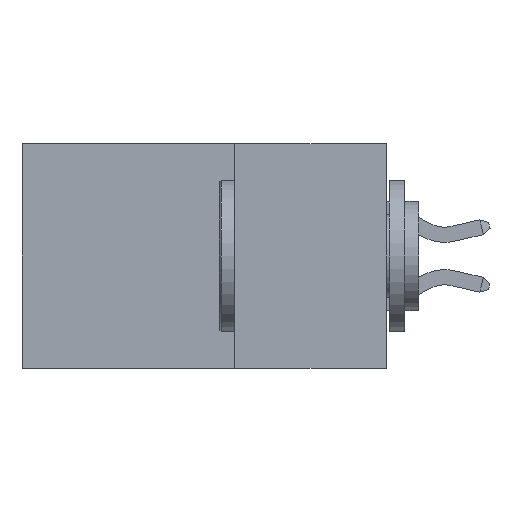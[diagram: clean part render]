
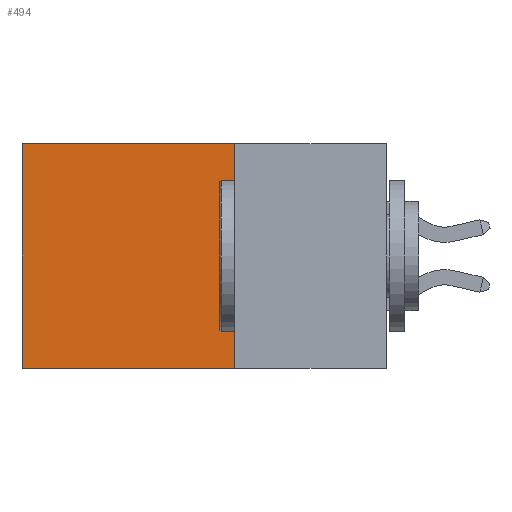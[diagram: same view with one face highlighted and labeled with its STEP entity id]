
A CAD part, left-side view. The second image highlights one B-rep face of the part: STEP entity #494.
In plain terms, the highlighted planar face has unit normal (-1, 0, 0).
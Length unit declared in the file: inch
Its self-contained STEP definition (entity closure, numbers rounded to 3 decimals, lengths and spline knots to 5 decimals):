
#291 = VECTOR ( 'NONE', #782, 39.37008 ) ;
#494 = ADVANCED_FACE ( 'NONE', ( #12663 ), #8164, .F. ) ;
#782 = DIRECTION ( 'NONE',  ( 0., 1., 0. ) ) ;
#1333 = VECTOR ( 'NONE', #10145, 39.37008 ) ;
#1853 = CARTESIAN_POINT ( 'NONE',  ( 0.298, 0.25, -0.37 ) ) ;
#2065 = VECTOR ( 'NONE', #10781, 39.37008 ) ;
#2215 = CARTESIAN_POINT ( 'NONE',  ( 0.298, 0.6, 0. ) ) ;
#2294 = EDGE_CURVE ( 'NONE', #17666, #16864, #17444, .T. ) ;
#3424 = CARTESIAN_POINT ( 'NONE',  ( 0.298, 0.6, -0.37 ) ) ;
#3430 = ORIENTED_EDGE ( 'NONE', *, *, #13129, .F. ) ;
#3435 = EDGE_CURVE ( 'NONE', #16864, #8720, #5317, .T. ) ;
#4284 = LINE ( 'NONE', #9667, #291 ) ;
#4537 = AXIS2_PLACEMENT_3D ( 'NONE', #12286, #16234, #17182 ) ;
#5317 = LINE ( 'NONE', #2215, #1333 ) ;
#5901 = ORIENTED_EDGE ( 'NONE', *, *, #8180, .F. ) ;
#7679 = CARTESIAN_POINT ( 'NONE',  ( 0.298, 0.25, 0. ) ) ;
#7924 = ORIENTED_EDGE ( 'NONE', *, *, #2294, .T. ) ;
#8071 = LINE ( 'NONE', #8319, #15497 ) ;
#8164 = PLANE ( 'NONE',  #4537 ) ;
#8180 = EDGE_CURVE ( 'NONE', #11720, #8720, #4284, .T. ) ;
#8319 = CARTESIAN_POINT ( 'NONE',  ( 0.298, 0.25, 0. ) ) ;
#8720 = VERTEX_POINT ( 'NONE', #3424 ) ;
#9667 = CARTESIAN_POINT ( 'NONE',  ( 0.298, 0.25, -0.37 ) ) ;
#9789 = DIRECTION ( 'NONE',  ( 0., 0., -1. ) ) ;
#10145 = DIRECTION ( 'NONE',  ( 0., 0., -1. ) ) ;
#10781 = DIRECTION ( 'NONE',  ( 0., 1., 0. ) ) ;
#11720 = VERTEX_POINT ( 'NONE', #1853 ) ;
#12286 = CARTESIAN_POINT ( 'NONE',  ( 0.298, 0.25, 0. ) ) ;
#12663 = FACE_OUTER_BOUND ( 'NONE', #13886, .T. ) ;
#13129 = EDGE_CURVE ( 'NONE', #17666, #11720, #8071, .T. ) ;
#13886 = EDGE_LOOP ( 'NONE', ( #14840, #5901, #3430, #7924 ) ) ;
#14840 = ORIENTED_EDGE ( 'NONE', *, *, #3435, .T. ) ;
#15497 = VECTOR ( 'NONE', #9789, 39.37008 ) ;
#16234 = DIRECTION ( 'NONE',  ( 1., 0., 0. ) ) ;
#16766 = CARTESIAN_POINT ( 'NONE',  ( 0.298, 0.25, 0. ) ) ;
#16864 = VERTEX_POINT ( 'NONE', #17314 ) ;
#17182 = DIRECTION ( 'NONE',  ( 0., 0., -1. ) ) ;
#17314 = CARTESIAN_POINT ( 'NONE',  ( 0.298, 0.6, 0. ) ) ;
#17444 = LINE ( 'NONE', #16766, #2065 ) ;
#17666 = VERTEX_POINT ( 'NONE', #7679 ) ;
